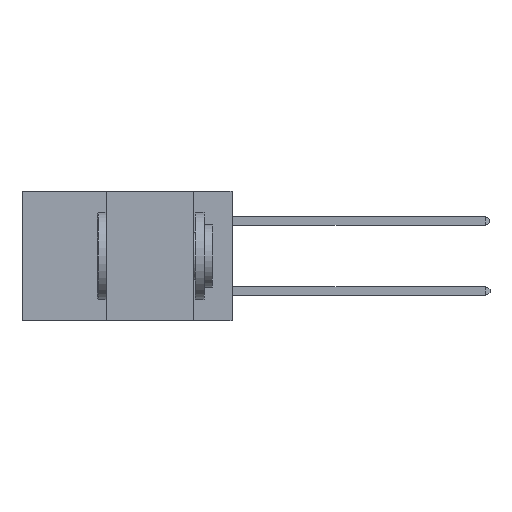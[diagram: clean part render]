
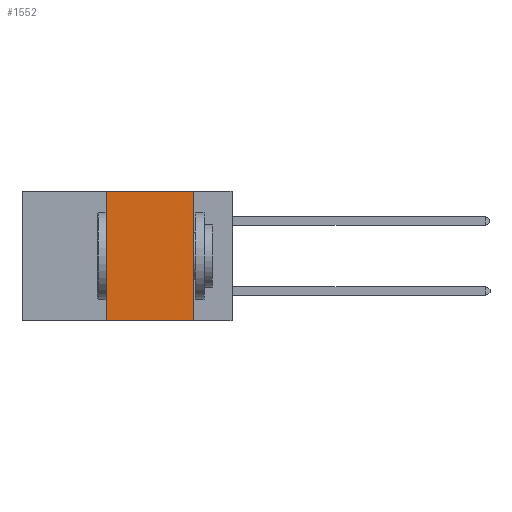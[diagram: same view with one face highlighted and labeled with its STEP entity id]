
A CAD part, left-side view. The second image highlights one B-rep face of the part: STEP entity #1552.
In plain terms, the highlighted planar face has unit normal (-1, 0, 0).
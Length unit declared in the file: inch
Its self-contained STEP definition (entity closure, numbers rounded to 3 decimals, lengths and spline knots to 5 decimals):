
#239 = ORIENTED_EDGE ( 'NONE', *, *, #14843, .F. ) ;
#644 = CARTESIAN_POINT ( 'NONE',  ( 0., 0.6, 0. ) ) ;
#843 = DIRECTION ( 'NONE',  ( 0., -1., 0. ) ) ;
#1329 = CARTESIAN_POINT ( 'NONE',  ( 0., 0.11, -0.37 ) ) ;
#1548 = DIRECTION ( 'NONE',  ( 0., 0., -1. ) ) ;
#1552 = ADVANCED_FACE ( 'NONE', ( #10887 ), #1918, .F. ) ;
#1682 = ORIENTED_EDGE ( 'NONE', *, *, #9444, .F. ) ;
#1918 = PLANE ( 'NONE',  #3054 ) ;
#2220 = DIRECTION ( 'NONE',  ( 1., 0., 0. ) ) ;
#2307 = ORIENTED_EDGE ( 'NONE', *, *, #12678, .T. ) ;
#2564 = DIRECTION ( 'NONE',  ( 0., -1., 0. ) ) ;
#3054 = AXIS2_PLACEMENT_3D ( 'NONE', #4775, #2220, #1548 ) ;
#3791 = VERTEX_POINT ( 'NONE', #21735 ) ;
#4698 = CARTESIAN_POINT ( 'NONE',  ( 0., 0.36, 0. ) ) ;
#4775 = CARTESIAN_POINT ( 'NONE',  ( 0., 0.6, 0. ) ) ;
#5637 = VECTOR ( 'NONE', #843, 39.37008 ) ;
#5900 = EDGE_CURVE ( 'NONE', #3791, #8649, #10707, .T. ) ;
#6389 = VECTOR ( 'NONE', #9931, 39.37008 ) ;
#6524 = CARTESIAN_POINT ( 'NONE',  ( 0., 0.6, -0.37 ) ) ;
#8075 = LINE ( 'NONE', #4698, #8619 ) ;
#8619 = VECTOR ( 'NONE', #15176, 39.37008 ) ;
#8649 = VERTEX_POINT ( 'NONE', #12722 ) ;
#9444 = EDGE_CURVE ( 'NONE', #15313, #3791, #8075, .T. ) ;
#9931 = DIRECTION ( 'NONE',  ( 0., 0., -1. ) ) ;
#10290 = ORIENTED_EDGE ( 'NONE', *, *, #5900, .F. ) ;
#10511 = LINE ( 'NONE', #20431, #6389 ) ;
#10707 = LINE ( 'NONE', #644, #14759 ) ;
#10887 = FACE_OUTER_BOUND ( 'NONE', #15732, .T. ) ;
#12678 = EDGE_CURVE ( 'NONE', #15313, #14401, #14910, .T. ) ;
#12722 = CARTESIAN_POINT ( 'NONE',  ( 0., 0.11, 0. ) ) ;
#13210 = CARTESIAN_POINT ( 'NONE',  ( 0., 0.36, -0.37 ) ) ;
#14401 = VERTEX_POINT ( 'NONE', #1329 ) ;
#14759 = VECTOR ( 'NONE', #2564, 39.37008 ) ;
#14843 = EDGE_CURVE ( 'NONE', #8649, #14401, #10511, .T. ) ;
#14910 = LINE ( 'NONE', #6524, #5637 ) ;
#15176 = DIRECTION ( 'NONE',  ( 0., 0., 1. ) ) ;
#15313 = VERTEX_POINT ( 'NONE', #13210 ) ;
#15732 = EDGE_LOOP ( 'NONE', ( #239, #10290, #1682, #2307 ) ) ;
#20431 = CARTESIAN_POINT ( 'NONE',  ( 0., 0.11, 0. ) ) ;
#21735 = CARTESIAN_POINT ( 'NONE',  ( 0., 0.36, 0. ) ) ;
